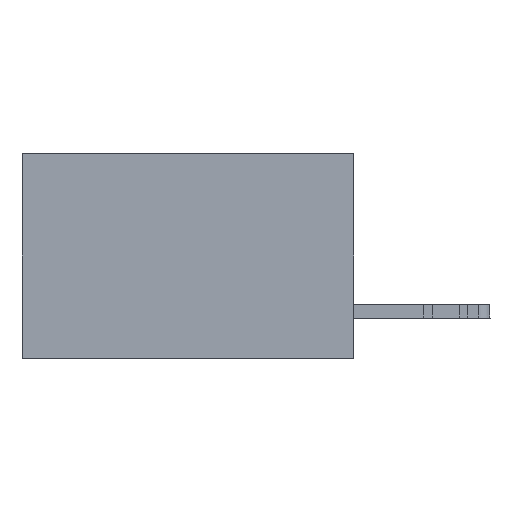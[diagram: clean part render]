
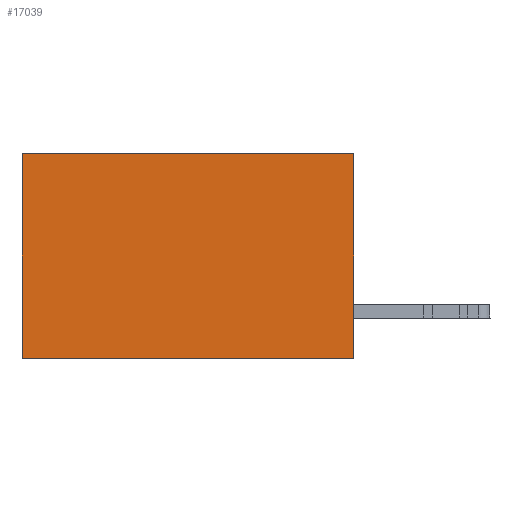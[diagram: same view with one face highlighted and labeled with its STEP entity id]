
A CAD part, left-side view. The second image highlights one B-rep face of the part: STEP entity #17039.
In plain terms, the highlighted planar face has unit normal (-1, 0, 0).
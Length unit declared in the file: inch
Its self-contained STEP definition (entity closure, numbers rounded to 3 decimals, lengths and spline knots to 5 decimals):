
#567 = EDGE_CURVE ( 'NONE', #4711, #41500, #35772, .T. ) ;
#995 = EDGE_CURVE ( 'NONE', #4711, #32007, #16608, .T. ) ;
#3086 = DIRECTION ( 'NONE',  ( 0., 0., -1. ) ) ;
#3286 = CARTESIAN_POINT ( 'NONE',  ( 0.2875, 0.6, -0.37 ) ) ;
#3559 = EDGE_CURVE ( 'NONE', #32007, #24679, #38270, .T. ) ;
#4359 = LINE ( 'NONE', #32742, #38710 ) ;
#4711 = VERTEX_POINT ( 'NONE', #19754 ) ;
#7524 = EDGE_LOOP ( 'NONE', ( #7676, #8307, #42368, #42293 ) ) ;
#7676 = ORIENTED_EDGE ( 'NONE', *, *, #24186, .T. ) ;
#8307 = ORIENTED_EDGE ( 'NONE', *, *, #3559, .F. ) ;
#9004 = AXIS2_PLACEMENT_3D ( 'NONE', #39434, #43017, #3086 ) ;
#9160 = DIRECTION ( 'NONE',  ( 0., 0., -1. ) ) ;
#9306 = CARTESIAN_POINT ( 'NONE',  ( 0.2875, 0., 0. ) ) ;
#16608 = LINE ( 'NONE', #9306, #21293 ) ;
#17039 = ADVANCED_FACE ( 'NONE', ( #35586 ), #29512, .F. ) ;
#17462 = DIRECTION ( 'NONE',  ( 0., 1., 0. ) ) ;
#19754 = CARTESIAN_POINT ( 'NONE',  ( 0.2875, 0., 0. ) ) ;
#21293 = VECTOR ( 'NONE', #9160, 39.37008 ) ;
#24186 = EDGE_CURVE ( 'NONE', #41500, #24679, #4359, .T. ) ;
#24679 = VERTEX_POINT ( 'NONE', #3286 ) ;
#26795 = CARTESIAN_POINT ( 'NONE',  ( 0.2875, 0., -0.37 ) ) ;
#26904 = VECTOR ( 'NONE', #17462, 39.37008 ) ;
#27031 = DIRECTION ( 'NONE',  ( 0., 1., 0. ) ) ;
#29394 = DIRECTION ( 'NONE',  ( 0., 0., -1. ) ) ;
#29512 = PLANE ( 'NONE',  #9004 ) ;
#30227 = CARTESIAN_POINT ( 'NONE',  ( 0.2875, 0., -0.37 ) ) ;
#30437 = VECTOR ( 'NONE', #27031, 39.37008 ) ;
#30462 = CARTESIAN_POINT ( 'NONE',  ( 0.2875, 0.6, 0. ) ) ;
#32007 = VERTEX_POINT ( 'NONE', #26795 ) ;
#32742 = CARTESIAN_POINT ( 'NONE',  ( 0.2875, 0.6, 0. ) ) ;
#35586 = FACE_OUTER_BOUND ( 'NONE', #7524, .T. ) ;
#35772 = LINE ( 'NONE', #36920, #26904 ) ;
#36920 = CARTESIAN_POINT ( 'NONE',  ( 0.2875, 0., 0. ) ) ;
#38270 = LINE ( 'NONE', #30227, #30437 ) ;
#38710 = VECTOR ( 'NONE', #29394, 39.37008 ) ;
#39434 = CARTESIAN_POINT ( 'NONE',  ( 0.2875, 0., 0. ) ) ;
#41500 = VERTEX_POINT ( 'NONE', #30462 ) ;
#42293 = ORIENTED_EDGE ( 'NONE', *, *, #567, .T. ) ;
#42368 = ORIENTED_EDGE ( 'NONE', *, *, #995, .F. ) ;
#43017 = DIRECTION ( 'NONE',  ( 1., 0., 0. ) ) ;
